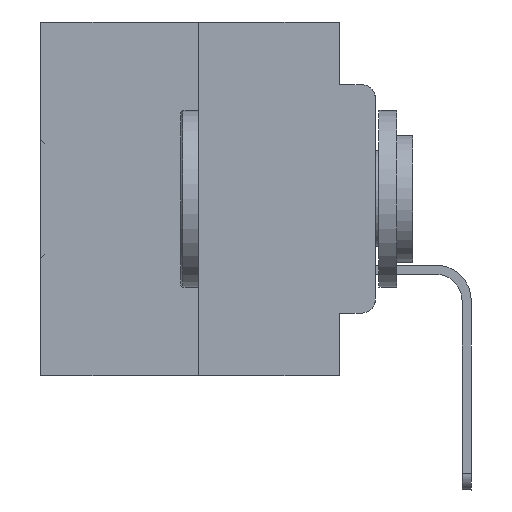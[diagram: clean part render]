
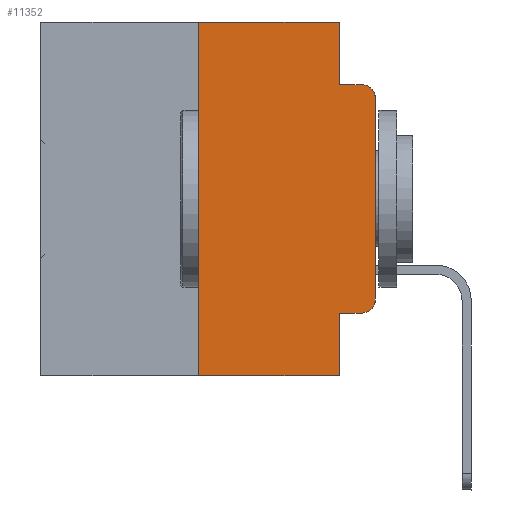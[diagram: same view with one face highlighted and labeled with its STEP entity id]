
A CAD part, left-side view. The second image highlights one B-rep face of the part: STEP entity #11352.
In plain terms, the highlighted planar face has unit normal (-1, 0, 0).
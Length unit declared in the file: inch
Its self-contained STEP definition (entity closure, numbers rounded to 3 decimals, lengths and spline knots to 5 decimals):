
#98 = FACE_OUTER_BOUND ( 'NONE', #15220, .T. ) ;
#341 = CARTESIAN_POINT ( 'NONE',  ( 0., 0.051, -0.4115 ) ) ;
#1213 = LINE ( 'NONE', #26094, #18602 ) ;
#1694 = DIRECTION ( 'NONE',  ( 0., 0., -1. ) ) ;
#1777 = EDGE_CURVE ( 'NONE', #25231, #31162, #5574, .T. ) ;
#2033 = DIRECTION ( 'NONE',  ( 0., -1., 0. ) ) ;
#2517 = EDGE_CURVE ( 'NONE', #11628, #18115, #1213, .T. ) ;
#2736 = VERTEX_POINT ( 'NONE', #29819 ) ;
#3358 = CIRCLE ( 'NONE', #31064, 0.02 ) ;
#3627 = DIRECTION ( 'NONE',  ( 0., 0., -1. ) ) ;
#3878 = VECTOR ( 'NONE', #21600, 39.37008 ) ;
#4046 = EDGE_CURVE ( 'NONE', #2736, #30870, #24395, .T. ) ;
#4249 = LINE ( 'NONE', #29650, #23210 ) ;
#5170 = ORIENTED_EDGE ( 'NONE', *, *, #10056, .T. ) ;
#5187 = CARTESIAN_POINT ( 'NONE',  ( 0., 0.25, -0.5 ) ) ;
#5574 = LINE ( 'NONE', #11030, #28941 ) ;
#6608 = VECTOR ( 'NONE', #32517, 39.37008 ) ;
#6929 = CARTESIAN_POINT ( 'NONE',  ( 0., 0.051, -0.4115 ) ) ;
#7146 = DIRECTION ( 'NONE',  ( 0., -1., 0. ) ) ;
#8377 = CARTESIAN_POINT ( 'NONE',  ( 0., 0., -0.1085 ) ) ;
#8434 = DIRECTION ( 'NONE',  ( -1., 0., 0. ) ) ;
#8502 = CARTESIAN_POINT ( 'NONE',  ( 0., 0.02, -0.1085 ) ) ;
#9118 = CARTESIAN_POINT ( 'NONE',  ( 0., 0.051, -0.0885 ) ) ;
#9223 = CARTESIAN_POINT ( 'NONE',  ( 0., 0.051, -0.0885 ) ) ;
#9428 = EDGE_CURVE ( 'NONE', #29920, #22131, #28707, .T. ) ;
#10056 = EDGE_CURVE ( 'NONE', #13899, #17325, #3358, .T. ) ;
#10298 = ORIENTED_EDGE ( 'NONE', *, *, #19672, .T. ) ;
#11030 = CARTESIAN_POINT ( 'NONE',  ( 0., 0.25, 0. ) ) ;
#11352 = ADVANCED_FACE ( 'NONE', ( #98 ), #26875, .F. ) ;
#11372 = ORIENTED_EDGE ( 'NONE', *, *, #19632, .F. ) ;
#11628 = VERTEX_POINT ( 'NONE', #341 ) ;
#11800 = LINE ( 'NONE', #6929, #29927 ) ;
#12056 = AXIS2_PLACEMENT_3D ( 'NONE', #32191, #22014, #1694 ) ;
#12136 = CARTESIAN_POINT ( 'NONE',  ( 0., 0., -0.3915 ) ) ;
#12197 = CARTESIAN_POINT ( 'NONE',  ( 0., 0.051, 0. ) ) ;
#12359 = EDGE_CURVE ( 'NONE', #11628, #29920, #11800, .T. ) ;
#13309 = DIRECTION ( 'NONE',  ( 0., 0., -1. ) ) ;
#13398 = DIRECTION ( 'NONE',  ( 0., -1., 0. ) ) ;
#13899 = VERTEX_POINT ( 'NONE', #8377 ) ;
#13936 = DIRECTION ( 'NONE',  ( -1., 0., 0. ) ) ;
#14179 = LINE ( 'NONE', #29120, #3878 ) ;
#15220 = EDGE_LOOP ( 'NONE', ( #10298, #5170, #11372, #19222, #22011, #22006, #25317, #32251, #28331, #25465 ) ) ;
#15292 = CARTESIAN_POINT ( 'NONE',  ( 0., 0.25, 0. ) ) ;
#15977 = CARTESIAN_POINT ( 'NONE',  ( 0., 0.02, -0.3915 ) ) ;
#17194 = CARTESIAN_POINT ( 'NONE',  ( 0., 0.02, -0.0885 ) ) ;
#17325 = VERTEX_POINT ( 'NONE', #17194 ) ;
#17407 = LINE ( 'NONE', #25846, #31669 ) ;
#18115 = VERTEX_POINT ( 'NONE', #23514 ) ;
#18602 = VECTOR ( 'NONE', #13309, 39.37008 ) ;
#19222 = ORIENTED_EDGE ( 'NONE', *, *, #4046, .F. ) ;
#19632 = EDGE_CURVE ( 'NONE', #30870, #17325, #20497, .T. ) ;
#19672 = EDGE_CURVE ( 'NONE', #22131, #13899, #14179, .T. ) ;
#20497 = LINE ( 'NONE', #9118, #23615 ) ;
#21364 = DIRECTION ( 'NONE',  ( 0., 0., -1. ) ) ;
#21523 = AXIS2_PLACEMENT_3D ( 'NONE', #15977, #8434, #21364 ) ;
#21600 = DIRECTION ( 'NONE',  ( 0., 0., 1. ) ) ;
#22006 = ORIENTED_EDGE ( 'NONE', *, *, #1777, .F. ) ;
#22011 = ORIENTED_EDGE ( 'NONE', *, *, #28994, .F. ) ;
#22014 = DIRECTION ( 'NONE',  ( 1., 0., 0. ) ) ;
#22131 = VERTEX_POINT ( 'NONE', #12136 ) ;
#23210 = VECTOR ( 'NONE', #2033, 39.37008 ) ;
#23514 = CARTESIAN_POINT ( 'NONE',  ( 0., 0.051, -0.5 ) ) ;
#23615 = VECTOR ( 'NONE', #29342, 39.37008 ) ;
#24395 = LINE ( 'NONE', #12197, #6608 ) ;
#25231 = VERTEX_POINT ( 'NONE', #5187 ) ;
#25317 = ORIENTED_EDGE ( 'NONE', *, *, #26698, .T. ) ;
#25465 = ORIENTED_EDGE ( 'NONE', *, *, #9428, .T. ) ;
#25846 = CARTESIAN_POINT ( 'NONE',  ( 0., 0.473, -0.5 ) ) ;
#26094 = CARTESIAN_POINT ( 'NONE',  ( 0., 0.051, 0. ) ) ;
#26698 = EDGE_CURVE ( 'NONE', #25231, #18115, #17407, .T. ) ;
#26875 = PLANE ( 'NONE',  #12056 ) ;
#28331 = ORIENTED_EDGE ( 'NONE', *, *, #12359, .T. ) ;
#28707 = CIRCLE ( 'NONE', #21523, 0.02 ) ;
#28941 = VECTOR ( 'NONE', #30791, 39.37008 ) ;
#28994 = EDGE_CURVE ( 'NONE', #31162, #2736, #4249, .T. ) ;
#29120 = CARTESIAN_POINT ( 'NONE',  ( 0., 0., 0. ) ) ;
#29342 = DIRECTION ( 'NONE',  ( 0., -1., 0. ) ) ;
#29650 = CARTESIAN_POINT ( 'NONE',  ( 0., 0.473, 0. ) ) ;
#29819 = CARTESIAN_POINT ( 'NONE',  ( 0., 0.051, 0. ) ) ;
#29920 = VERTEX_POINT ( 'NONE', #32683 ) ;
#29927 = VECTOR ( 'NONE', #7146, 39.37008 ) ;
#30791 = DIRECTION ( 'NONE',  ( 0., 0., 1. ) ) ;
#30870 = VERTEX_POINT ( 'NONE', #9223 ) ;
#31064 = AXIS2_PLACEMENT_3D ( 'NONE', #8502, #13936, #3627 ) ;
#31162 = VERTEX_POINT ( 'NONE', #15292 ) ;
#31669 = VECTOR ( 'NONE', #13398, 39.37008 ) ;
#32191 = CARTESIAN_POINT ( 'NONE',  ( 0., 0.473, 0. ) ) ;
#32251 = ORIENTED_EDGE ( 'NONE', *, *, #2517, .F. ) ;
#32517 = DIRECTION ( 'NONE',  ( 0., 0., -1. ) ) ;
#32683 = CARTESIAN_POINT ( 'NONE',  ( 0., 0.02, -0.4115 ) ) ;
